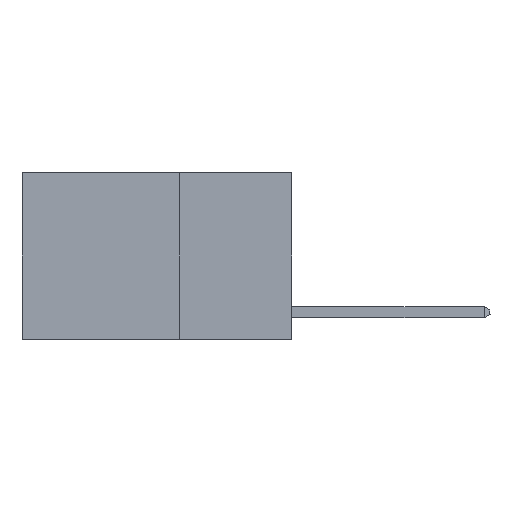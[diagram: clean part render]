
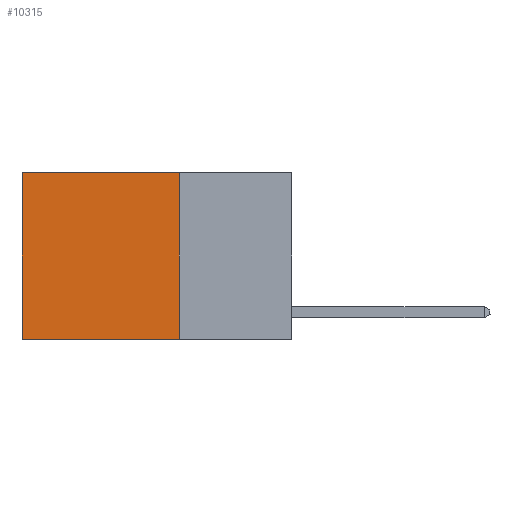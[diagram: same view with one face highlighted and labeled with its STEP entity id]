
A CAD part, left-side view. The second image highlights one B-rep face of the part: STEP entity #10315.
In plain terms, the highlighted planar face has unit normal (-1, 0, 0).
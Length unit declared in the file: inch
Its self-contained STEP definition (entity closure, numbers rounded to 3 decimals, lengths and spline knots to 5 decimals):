
#106 = EDGE_CURVE ( 'NONE', #1993, #9830, #1380, .T. ) ;
#608 = ORIENTED_EDGE ( 'NONE', *, *, #11638, .T. ) ;
#632 = DIRECTION ( 'NONE',  ( 1., 0., 0. ) ) ;
#723 = DIRECTION ( 'NONE',  ( 0., 1., 0. ) ) ;
#993 = VECTOR ( 'NONE', #3780, 39.37008 ) ;
#1120 = FACE_OUTER_BOUND ( 'NONE', #14817, .T. ) ;
#1380 = LINE ( 'NONE', #20002, #19413 ) ;
#1993 = VERTEX_POINT ( 'NONE', #20545 ) ;
#3780 = DIRECTION ( 'NONE',  ( 0., 1., 0. ) ) ;
#4451 = ORIENTED_EDGE ( 'NONE', *, *, #17023, .F. ) ;
#4700 = AXIS2_PLACEMENT_3D ( 'NONE', #10232, #632, #11839 ) ;
#5403 = CARTESIAN_POINT ( 'NONE',  ( 0.2625, 0.25, -0.37 ) ) ;
#7003 = PLANE ( 'NONE',  #4700 ) ;
#8649 = VERTEX_POINT ( 'NONE', #13992 ) ;
#9830 = VERTEX_POINT ( 'NONE', #10533 ) ;
#9832 = ORIENTED_EDGE ( 'NONE', *, *, #106, .T. ) ;
#10120 = ORIENTED_EDGE ( 'NONE', *, *, #12953, .F. ) ;
#10232 = CARTESIAN_POINT ( 'NONE',  ( 0.2625, 0.25, 0. ) ) ;
#10315 = ADVANCED_FACE ( 'NONE', ( #1120 ), #7003, .F. ) ;
#10533 = CARTESIAN_POINT ( 'NONE',  ( 0.2625, 0.6, -0.37 ) ) ;
#11638 = EDGE_CURVE ( 'NONE', #13803, #1993, #13297, .T. ) ;
#11839 = DIRECTION ( 'NONE',  ( 0., 0., -1. ) ) ;
#12310 = VECTOR ( 'NONE', #723, 39.37008 ) ;
#12953 = EDGE_CURVE ( 'NONE', #8649, #9830, #18339, .T. ) ;
#13297 = LINE ( 'NONE', #19919, #12310 ) ;
#13803 = VERTEX_POINT ( 'NONE', #18762 ) ;
#13992 = CARTESIAN_POINT ( 'NONE',  ( 0.2625, 0.25, -0.37 ) ) ;
#14569 = DIRECTION ( 'NONE',  ( 0., 0., -1. ) ) ;
#14817 = EDGE_LOOP ( 'NONE', ( #9832, #10120, #4451, #608 ) ) ;
#16162 = VECTOR ( 'NONE', #14569, 39.37008 ) ;
#17023 = EDGE_CURVE ( 'NONE', #13803, #8649, #20392, .T. ) ;
#18339 = LINE ( 'NONE', #5403, #993 ) ;
#18762 = CARTESIAN_POINT ( 'NONE',  ( 0.2625, 0.25, 0. ) ) ;
#19413 = VECTOR ( 'NONE', #20028, 39.37008 ) ;
#19919 = CARTESIAN_POINT ( 'NONE',  ( 0.2625, 0.25, 0. ) ) ;
#20002 = CARTESIAN_POINT ( 'NONE',  ( 0.2625, 0.6, 0. ) ) ;
#20028 = DIRECTION ( 'NONE',  ( 0., 0., -1. ) ) ;
#20392 = LINE ( 'NONE', #20645, #16162 ) ;
#20545 = CARTESIAN_POINT ( 'NONE',  ( 0.2625, 0.6, 0. ) ) ;
#20645 = CARTESIAN_POINT ( 'NONE',  ( 0.2625, 0.25, 0. ) ) ;
